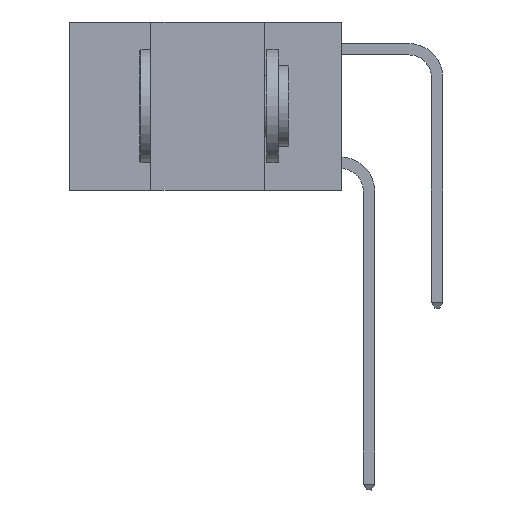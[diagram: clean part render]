
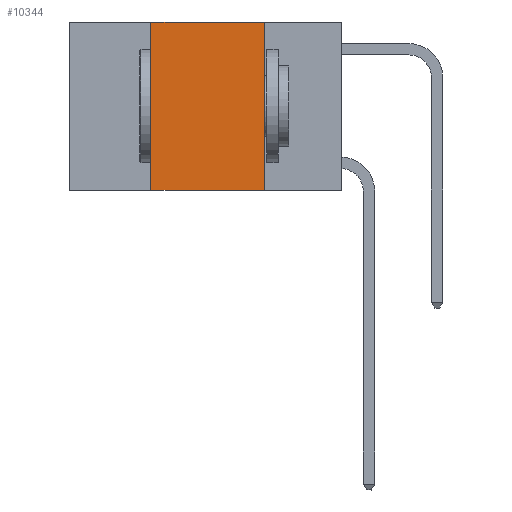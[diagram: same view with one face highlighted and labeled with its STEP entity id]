
A CAD part, left-side view. The second image highlights one B-rep face of the part: STEP entity #10344.
In plain terms, the highlighted planar face has unit normal (-1, 0, 0).
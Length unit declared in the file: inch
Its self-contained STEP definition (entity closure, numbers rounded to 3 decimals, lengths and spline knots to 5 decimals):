
#694 = LINE ( 'NONE', #30867, #13775 ) ;
#2395 = EDGE_CURVE ( 'NONE', #3781, #18715, #20613, .T. ) ;
#2644 = ORIENTED_EDGE ( 'NONE', *, *, #12100, .T. ) ;
#3748 = DIRECTION ( 'NONE',  ( 0., 0., -1. ) ) ;
#3781 = VERTEX_POINT ( 'NONE', #30602 ) ;
#6295 = CARTESIAN_POINT ( 'NONE',  ( 0., 0.42, -0.37 ) ) ;
#6998 = AXIS2_PLACEMENT_3D ( 'NONE', #29703, #19392, #3748 ) ;
#7158 = ORIENTED_EDGE ( 'NONE', *, *, #13912, .F. ) ;
#9996 = CARTESIAN_POINT ( 'NONE',  ( 0., 0.17, 0. ) ) ;
#10344 = ADVANCED_FACE ( 'NONE', ( #26970 ), #32265, .F. ) ;
#10492 = LINE ( 'NONE', #10518, #16584 ) ;
#10518 = CARTESIAN_POINT ( 'NONE',  ( 0., 0.42, 0. ) ) ;
#12100 = EDGE_CURVE ( 'NONE', #17007, #32013, #17890, .T. ) ;
#13662 = ORIENTED_EDGE ( 'NONE', *, *, #20914, .F. ) ;
#13775 = VECTOR ( 'NONE', #15353, 39.37008 ) ;
#13888 = CARTESIAN_POINT ( 'NONE',  ( 0., 0.17, -0.37 ) ) ;
#13912 = EDGE_CURVE ( 'NONE', #18715, #32013, #694, .T. ) ;
#15316 = ORIENTED_EDGE ( 'NONE', *, *, #2395, .F. ) ;
#15353 = DIRECTION ( 'NONE',  ( 0., 0., -1. ) ) ;
#16584 = VECTOR ( 'NONE', #21021, 39.37008 ) ;
#17007 = VERTEX_POINT ( 'NONE', #6295 ) ;
#17371 = EDGE_LOOP ( 'NONE', ( #7158, #15316, #13662, #2644 ) ) ;
#17890 = LINE ( 'NONE', #26796, #30858 ) ;
#18715 = VERTEX_POINT ( 'NONE', #9996 ) ;
#19392 = DIRECTION ( 'NONE',  ( 1., 0., 0. ) ) ;
#20613 = LINE ( 'NONE', #23133, #27476 ) ;
#20914 = EDGE_CURVE ( 'NONE', #17007, #3781, #10492, .T. ) ;
#21021 = DIRECTION ( 'NONE',  ( 0., 0., 1. ) ) ;
#23133 = CARTESIAN_POINT ( 'NONE',  ( 0., 0.6, 0. ) ) ;
#26796 = CARTESIAN_POINT ( 'NONE',  ( 0., 0.6, -0.37 ) ) ;
#26970 = FACE_OUTER_BOUND ( 'NONE', #17371, .T. ) ;
#27476 = VECTOR ( 'NONE', #33253, 39.37008 ) ;
#29703 = CARTESIAN_POINT ( 'NONE',  ( 0., 0.6, 0. ) ) ;
#30602 = CARTESIAN_POINT ( 'NONE',  ( 0., 0.42, 0. ) ) ;
#30858 = VECTOR ( 'NONE', #31954, 39.37008 ) ;
#30867 = CARTESIAN_POINT ( 'NONE',  ( 0., 0.17, 0. ) ) ;
#31954 = DIRECTION ( 'NONE',  ( 0., -1., 0. ) ) ;
#32013 = VERTEX_POINT ( 'NONE', #13888 ) ;
#32265 = PLANE ( 'NONE',  #6998 ) ;
#33253 = DIRECTION ( 'NONE',  ( 0., -1., 0. ) ) ;
